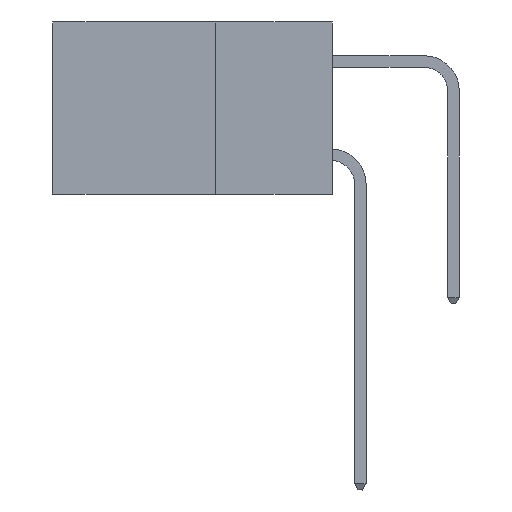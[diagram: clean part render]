
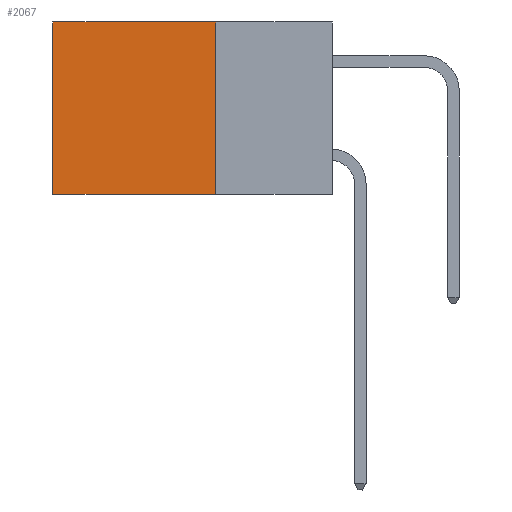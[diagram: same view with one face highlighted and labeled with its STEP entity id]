
A CAD part, left-side view. The second image highlights one B-rep face of the part: STEP entity #2067.
In plain terms, the highlighted planar face has unit normal (-1, 0, 0).
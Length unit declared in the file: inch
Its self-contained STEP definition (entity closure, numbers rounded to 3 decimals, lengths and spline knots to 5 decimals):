
#149 = CARTESIAN_POINT ( 'NONE',  ( 0.298, 0.25, 0. ) ) ;
#919 = EDGE_CURVE ( 'NONE', #30983, #22401, #5717, .T. ) ;
#2067 = ADVANCED_FACE ( 'NONE', ( #9957 ), #15969, .F. ) ;
#2924 = CARTESIAN_POINT ( 'NONE',  ( 0.298, 0.25, -0.37 ) ) ;
#3547 = LINE ( 'NONE', #30634, #8257 ) ;
#3640 = LINE ( 'NONE', #2924, #17785 ) ;
#3946 = CARTESIAN_POINT ( 'NONE',  ( 0.298, 0.6, 0. ) ) ;
#4494 = ORIENTED_EDGE ( 'NONE', *, *, #19662, .F. ) ;
#4983 = AXIS2_PLACEMENT_3D ( 'NONE', #149, #25138, #16458 ) ;
#5717 = LINE ( 'NONE', #6673, #26834 ) ;
#5783 = DIRECTION ( 'NONE',  ( 0., 1., 0. ) ) ;
#6432 = DIRECTION ( 'NONE',  ( 0., 0., -1. ) ) ;
#6673 = CARTESIAN_POINT ( 'NONE',  ( 0.298, 0.6, 0. ) ) ;
#7393 = CARTESIAN_POINT ( 'NONE',  ( 0.298, 0.25, 0. ) ) ;
#8041 = EDGE_CURVE ( 'NONE', #8123, #17368, #10939, .T. ) ;
#8123 = VERTEX_POINT ( 'NONE', #7393 ) ;
#8257 = VECTOR ( 'NONE', #19677, 39.37008 ) ;
#9402 = CARTESIAN_POINT ( 'NONE',  ( 0.298, 0.6, -0.37 ) ) ;
#9669 = CARTESIAN_POINT ( 'NONE',  ( 0.298, 0.25, 0. ) ) ;
#9957 = FACE_OUTER_BOUND ( 'NONE', #13629, .T. ) ;
#10939 = LINE ( 'NONE', #9669, #29412 ) ;
#13629 = EDGE_LOOP ( 'NONE', ( #23039, #4494, #24327, #14566 ) ) ;
#14566 = ORIENTED_EDGE ( 'NONE', *, *, #20949, .T. ) ;
#15969 = PLANE ( 'NONE',  #4983 ) ;
#16458 = DIRECTION ( 'NONE',  ( 0., 0., -1. ) ) ;
#17368 = VERTEX_POINT ( 'NONE', #24861 ) ;
#17785 = VECTOR ( 'NONE', #5783, 39.37008 ) ;
#19662 = EDGE_CURVE ( 'NONE', #17368, #22401, #3640, .T. ) ;
#19677 = DIRECTION ( 'NONE',  ( 0., 1., 0. ) ) ;
#20949 = EDGE_CURVE ( 'NONE', #8123, #30983, #3547, .T. ) ;
#22401 = VERTEX_POINT ( 'NONE', #9402 ) ;
#23039 = ORIENTED_EDGE ( 'NONE', *, *, #919, .T. ) ;
#23639 = DIRECTION ( 'NONE',  ( 0., 0., -1. ) ) ;
#24327 = ORIENTED_EDGE ( 'NONE', *, *, #8041, .F. ) ;
#24861 = CARTESIAN_POINT ( 'NONE',  ( 0.298, 0.25, -0.37 ) ) ;
#25138 = DIRECTION ( 'NONE',  ( 1., 0., 0. ) ) ;
#26834 = VECTOR ( 'NONE', #6432, 39.37008 ) ;
#29412 = VECTOR ( 'NONE', #23639, 39.37008 ) ;
#30634 = CARTESIAN_POINT ( 'NONE',  ( 0.298, 0.25, 0. ) ) ;
#30983 = VERTEX_POINT ( 'NONE', #3946 ) ;
